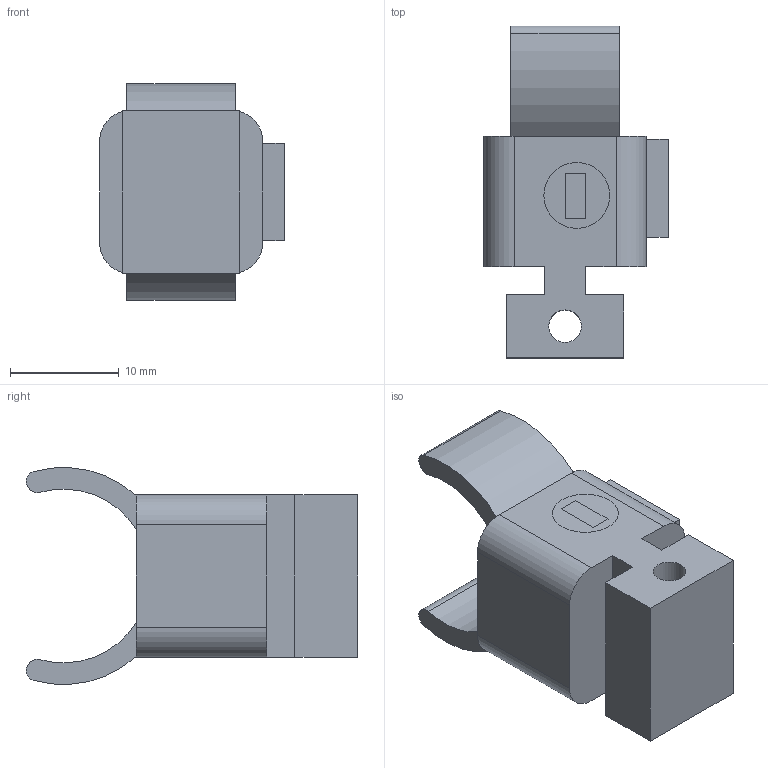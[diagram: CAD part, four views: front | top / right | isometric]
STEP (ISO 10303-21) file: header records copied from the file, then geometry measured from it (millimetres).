
FILE_DESCRIPTION(('FreeCAD Model'),'2;1');
FILE_NAME( 'sight post.step', '2018-04-06T19:15:43',('Author'),(''), 'Open CASCADE STEP processor 6.8','FreeCAD','Unknown');
FILE_SCHEMA(('AUTOMOTIVE_DESIGN_CC2 { 1 2 10303 214 -1 1 5 4 }'));
Length unit declared in the file: millimetre
Products named in the file (1): Fillet001
Bounding box: 17 x 30.55 x 19.96 mm (x, y, z)
Volume: 3680.2 mm3; surface area: 2714.8 mm2
Topology: 1 solids, 1 shells, 46 faces, 119 edges, 81 vertices
Faces by surface type: plane 30, cylinder 12, bspline 4
Full cylindrical faces by diameter (mm): 2.4 x1, 3 x1
Entity records: 5419 total; most frequent: CARTESIAN_POINT 3099, DIRECTION 395, LINE 250, VECTOR 250, ORIENTED_EDGE 238, PCURVE 238, DEFINITIONAL_REPRESENTATION 238, EDGE_CURVE 119
